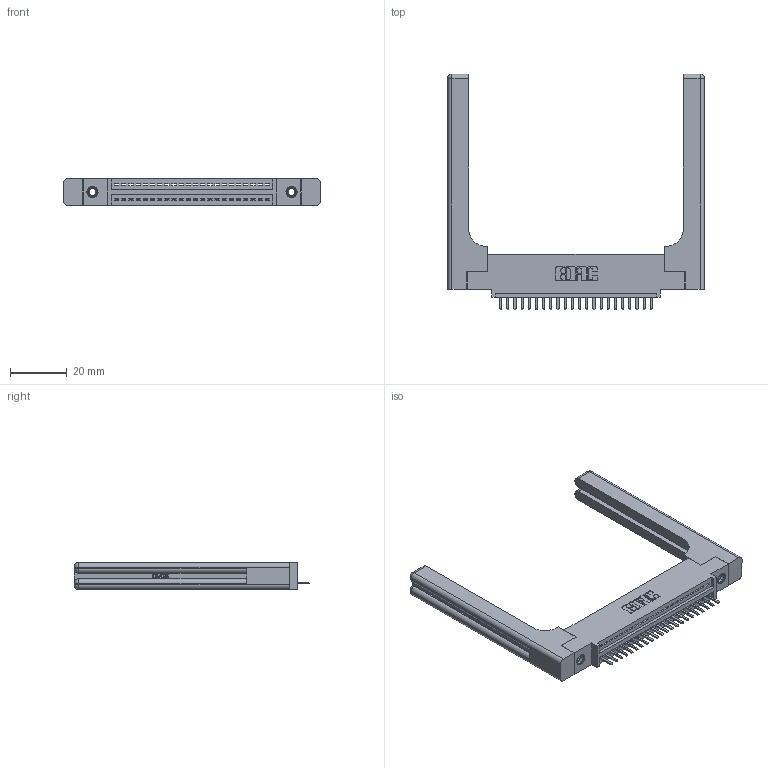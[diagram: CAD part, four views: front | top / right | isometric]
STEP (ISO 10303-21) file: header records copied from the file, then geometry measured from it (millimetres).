
FILE_DESCRIPTION (( 'STEP AP203' ), '1' );
FILE_NAME ('395-022-520-458.STEP', '2019-10-18T02:41:19', ( '' ), ( '' ), 'SwSTEP 2.0', 'SolidWorks 2016', '' );
FILE_SCHEMA (( 'CONFIG_CONTROL_DESIGN' ));
Length unit declared in the file: inch
Products named in the file (5): 395-022-520-458; 345-292-001_345-293-120; 345 Part_0.110 Offset - 0.156 Dia-TH; 345-220-058_345-220-058; 345-250-001_345-250-001-102
Assembly tree (27 placements, depth 2):
  395-022-520-458
    345 Part_0.110 Offset - 0.156 Dia-TH
    345-292-001_345-293-120  x22
    345-250-001_345-250-001-102  x2
    345-220-058_345-220-058  x2
Bounding box: 90.91 x 83.44 x 9.4 mm (x, y, z)
Volume: 16838.9 mm3; surface area: 15983.6 mm2
Topology: 27 solids, 27 shells, 1750 faces, 5067 edges, 3298 vertices
Faces by surface type: plane 1156, cylinder 534, bspline 36, cone 12, sphere 8, torus 4
Entity records: 24678 total; most frequent: CARTESIAN_POINT 5259, ORIENTED_EDGE 4000, DIRECTION 3556, EDGE_CURVE 2000, VECTOR 1684, LINE 1684, VERTEX_POINT 1322, AXIS2_PLACEMENT_3D 936
